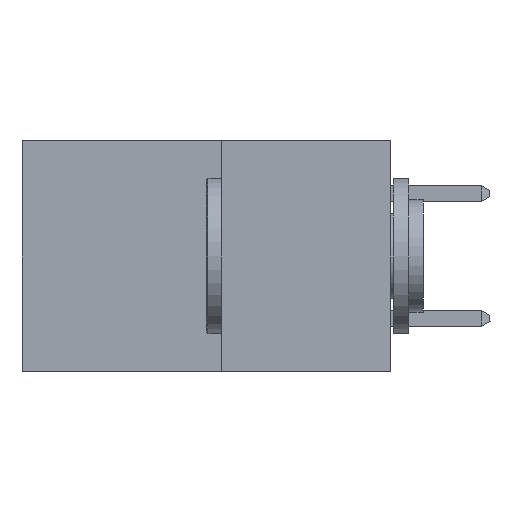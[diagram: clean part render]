
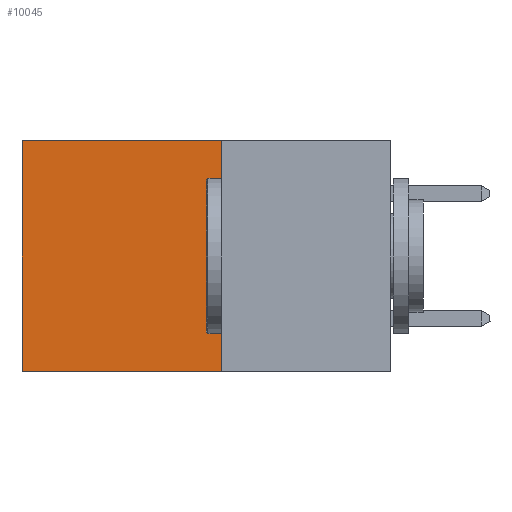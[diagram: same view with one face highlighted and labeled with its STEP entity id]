
A CAD part, left-side view. The second image highlights one B-rep face of the part: STEP entity #10045.
In plain terms, the highlighted planar face has unit normal (-1, 0, 0).
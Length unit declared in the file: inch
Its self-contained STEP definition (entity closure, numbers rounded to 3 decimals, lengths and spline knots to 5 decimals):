
#993 = VECTOR ( 'NONE', #3659, 39.37008 ) ;
#1672 = DIRECTION ( 'NONE',  ( 0., 0., -1. ) ) ;
#1808 = CARTESIAN_POINT ( 'NONE',  ( 0.277, 0.59, -0.37 ) ) ;
#2321 = CARTESIAN_POINT ( 'NONE',  ( 0.277, 0.27, 0. ) ) ;
#2738 = LINE ( 'NONE', #2321, #16927 ) ;
#3659 = DIRECTION ( 'NONE',  ( 0., 0., -1. ) ) ;
#3857 = ORIENTED_EDGE ( 'NONE', *, *, #14343, .F. ) ;
#4177 = DIRECTION ( 'NONE',  ( 0., 1., 0. ) ) ;
#4483 = EDGE_CURVE ( 'NONE', #18832, #14165, #10859, .T. ) ;
#4586 = LINE ( 'NONE', #21315, #23716 ) ;
#4751 = DIRECTION ( 'NONE',  ( 0., 1., 0. ) ) ;
#4913 = CARTESIAN_POINT ( 'NONE',  ( 0.277, 0.59, -0.37 ) ) ;
#4961 = DIRECTION ( 'NONE',  ( 0., 0., -1. ) ) ;
#5444 = AXIS2_PLACEMENT_3D ( 'NONE', #10472, #16034, #4961 ) ;
#8611 = ORIENTED_EDGE ( 'NONE', *, *, #4483, .T. ) ;
#8732 = CARTESIAN_POINT ( 'NONE',  ( 0.277, 0.27, 0. ) ) ;
#9526 = VERTEX_POINT ( 'NONE', #17978 ) ;
#10045 = ADVANCED_FACE ( 'NONE', ( #15365 ), #15962, .F. ) ;
#10472 = CARTESIAN_POINT ( 'NONE',  ( 0.277, 0.27, -0.37 ) ) ;
#10859 = LINE ( 'NONE', #1808, #993 ) ;
#11231 = EDGE_CURVE ( 'NONE', #9526, #14165, #4586, .T. ) ;
#12578 = LINE ( 'NONE', #16490, #17503 ) ;
#13412 = EDGE_LOOP ( 'NONE', ( #8611, #16303, #3857, #22442 ) ) ;
#14165 = VERTEX_POINT ( 'NONE', #4913 ) ;
#14343 = EDGE_CURVE ( 'NONE', #20882, #9526, #12578, .T. ) ;
#15365 = FACE_OUTER_BOUND ( 'NONE', #13412, .T. ) ;
#15962 = PLANE ( 'NONE',  #5444 ) ;
#16034 = DIRECTION ( 'NONE',  ( 1., 0., 0. ) ) ;
#16303 = ORIENTED_EDGE ( 'NONE', *, *, #11231, .F. ) ;
#16490 = CARTESIAN_POINT ( 'NONE',  ( 0.277, 0.27, -0.37 ) ) ;
#16927 = VECTOR ( 'NONE', #4177, 39.37008 ) ;
#17092 = EDGE_CURVE ( 'NONE', #20882, #18832, #2738, .T. ) ;
#17503 = VECTOR ( 'NONE', #1672, 39.37008 ) ;
#17978 = CARTESIAN_POINT ( 'NONE',  ( 0.277, 0.27, -0.37 ) ) ;
#18832 = VERTEX_POINT ( 'NONE', #20445 ) ;
#20445 = CARTESIAN_POINT ( 'NONE',  ( 0.277, 0.59, 0. ) ) ;
#20882 = VERTEX_POINT ( 'NONE', #8732 ) ;
#21315 = CARTESIAN_POINT ( 'NONE',  ( 0.277, 0.27, -0.37 ) ) ;
#22442 = ORIENTED_EDGE ( 'NONE', *, *, #17092, .T. ) ;
#23716 = VECTOR ( 'NONE', #4751, 39.37008 ) ;
